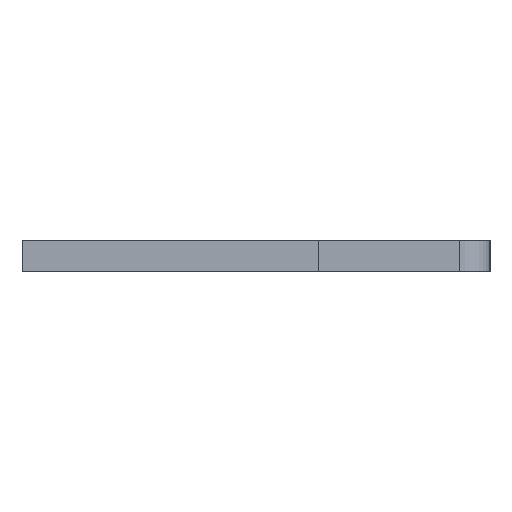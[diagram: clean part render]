
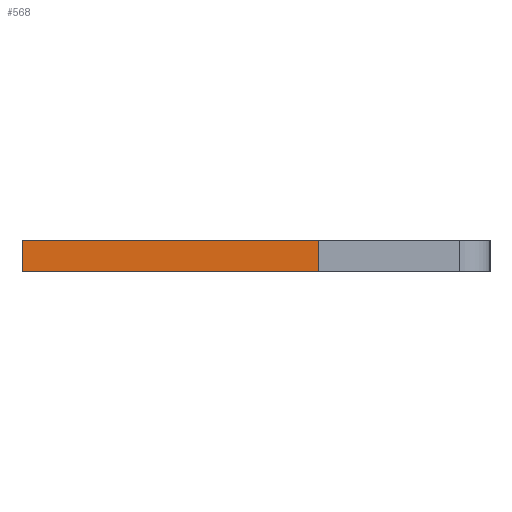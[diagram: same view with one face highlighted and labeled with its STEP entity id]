
A CAD part, left-side view. The second image highlights one B-rep face of the part: STEP entity #568.
In plain terms, the highlighted face is planar.
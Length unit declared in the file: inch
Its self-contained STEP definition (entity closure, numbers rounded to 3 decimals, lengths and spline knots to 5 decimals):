
#44 = DIRECTION ( 'NONE',  ( -1., 0., 0. ) ) ;
#62 = CARTESIAN_POINT ( 'NONE',  ( 0.01, 0.15, -0.04 ) ) ;
#306 = EDGE_LOOP ( 'NONE', ( #1466, #1967, #941, #2291 ) ) ;
#478 = CARTESIAN_POINT ( 'NONE',  ( 0.01, 0.15, -0.04 ) ) ;
#518 = DIRECTION ( 'NONE',  ( 0., 1., 0. ) ) ;
#561 = VERTEX_POINT ( 'NONE', #1491 ) ;
#568 = ADVANCED_FACE ( 'NONE', ( #1530 ), #891, .F. ) ;
#726 = VECTOR ( 'NONE', #818, 39.37008 ) ;
#808 = VECTOR ( 'NONE', #2080, 39.37008 ) ;
#818 = DIRECTION ( 'NONE',  ( -1., 0., 0. ) ) ;
#891 = PLANE ( 'NONE',  #2293 ) ;
#941 = ORIENTED_EDGE ( 'NONE', *, *, #2122, .F. ) ;
#948 = VECTOR ( 'NONE', #44, 39.37008 ) ;
#1053 = VERTEX_POINT ( 'NONE', #1311 ) ;
#1092 = DIRECTION ( 'NONE',  ( 0., 0., 1. ) ) ;
#1185 = EDGE_CURVE ( 'NONE', #1558, #561, #1319, .T. ) ;
#1305 = CARTESIAN_POINT ( 'NONE',  ( -0.01, -0.04, -0.04 ) ) ;
#1308 = VECTOR ( 'NONE', #518, 39.37008 ) ;
#1311 = CARTESIAN_POINT ( 'NONE',  ( 0.01, 0.15, -0.04 ) ) ;
#1319 = LINE ( 'NONE', #2036, #808 ) ;
#1466 = ORIENTED_EDGE ( 'NONE', *, *, #1185, .T. ) ;
#1491 = CARTESIAN_POINT ( 'NONE',  ( -0.01, 0.15, -0.04 ) ) ;
#1530 = FACE_OUTER_BOUND ( 'NONE', #306, .T. ) ;
#1558 = VERTEX_POINT ( 'NONE', #1305 ) ;
#1688 = CARTESIAN_POINT ( 'NONE',  ( 0.01, -0.04, -0.04 ) ) ;
#1704 = LINE ( 'NONE', #478, #948 ) ;
#1799 = EDGE_CURVE ( 'NONE', #1053, #561, #1704, .T. ) ;
#1967 = ORIENTED_EDGE ( 'NONE', *, *, #1799, .F. ) ;
#2036 = CARTESIAN_POINT ( 'NONE',  ( -0.01, 0.15, -0.04 ) ) ;
#2052 = DIRECTION ( 'NONE',  ( 1., 0., 0. ) ) ;
#2080 = DIRECTION ( 'NONE',  ( 0., 1., 0. ) ) ;
#2122 = EDGE_CURVE ( 'NONE', #2648, #1053, #2730, .T. ) ;
#2291 = ORIENTED_EDGE ( 'NONE', *, *, #2936, .T. ) ;
#2293 = AXIS2_PLACEMENT_3D ( 'NONE', #2494, #1092, #2052 ) ;
#2476 = LINE ( 'NONE', #2931, #726 ) ;
#2494 = CARTESIAN_POINT ( 'NONE',  ( 0.01, 0.15, -0.04 ) ) ;
#2648 = VERTEX_POINT ( 'NONE', #1688 ) ;
#2730 = LINE ( 'NONE', #62, #1308 ) ;
#2931 = CARTESIAN_POINT ( 'NONE',  ( 0.01, -0.04, -0.04 ) ) ;
#2936 = EDGE_CURVE ( 'NONE', #2648, #1558, #2476, .T. ) ;
